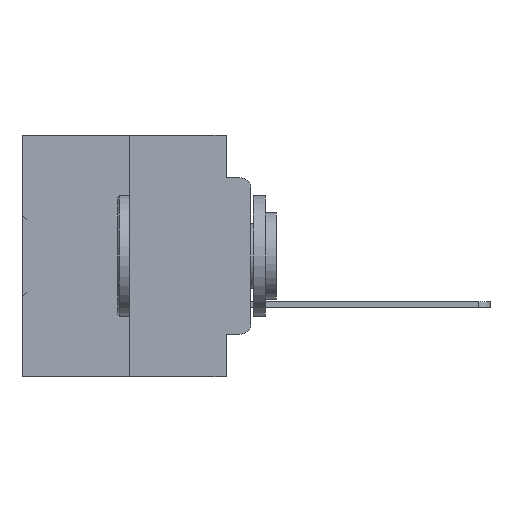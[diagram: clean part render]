
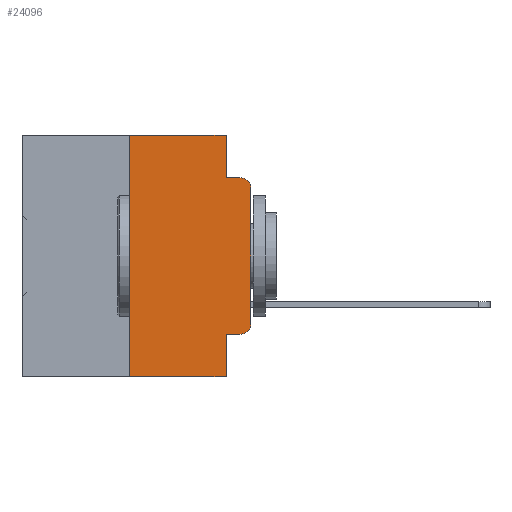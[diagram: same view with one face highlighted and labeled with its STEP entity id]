
A CAD part, left-side view. The second image highlights one B-rep face of the part: STEP entity #24096.
In plain terms, the highlighted planar face has unit normal (-1, 0, 0).
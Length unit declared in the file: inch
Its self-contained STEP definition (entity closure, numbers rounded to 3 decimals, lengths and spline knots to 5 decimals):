
#354 = DIRECTION ( 'NONE',  ( 0., 0., -1. ) ) ;
#585 = ORIENTED_EDGE ( 'NONE', *, *, #23253, .F. ) ;
#699 = EDGE_CURVE ( 'NONE', #13239, #17577, #24076, .T. ) ;
#1765 = ORIENTED_EDGE ( 'NONE', *, *, #35002, .F. ) ;
#1872 = ORIENTED_EDGE ( 'NONE', *, *, #27103, .F. ) ;
#2920 = VERTEX_POINT ( 'NONE', #25099 ) ;
#3272 = ORIENTED_EDGE ( 'NONE', *, *, #11423, .T. ) ;
#3606 = LINE ( 'NONE', #4797, #32485 ) ;
#4033 = CIRCLE ( 'NONE', #13072, 0.02 ) ;
#4127 = ORIENTED_EDGE ( 'NONE', *, *, #17073, .T. ) ;
#4234 = CARTESIAN_POINT ( 'NONE',  ( 0., 0.051, -0.0885 ) ) ;
#4304 = VERTEX_POINT ( 'NONE', #31393 ) ;
#4423 = VERTEX_POINT ( 'NONE', #23908 ) ;
#4560 = CARTESIAN_POINT ( 'NONE',  ( 0., 0.473, 0. ) ) ;
#4667 = VERTEX_POINT ( 'NONE', #35616 ) ;
#4797 = CARTESIAN_POINT ( 'NONE',  ( 0., 0.051, 0. ) ) ;
#4916 = ORIENTED_EDGE ( 'NONE', *, *, #32068, .F. ) ;
#5108 = ORIENTED_EDGE ( 'NONE', *, *, #699, .T. ) ;
#5327 = DIRECTION ( 'NONE',  ( -1., 0., 0. ) ) ;
#6555 = LINE ( 'NONE', #34905, #35234 ) ;
#7969 = CARTESIAN_POINT ( 'NONE',  ( 0., 0.25, -0.5 ) ) ;
#8515 = ORIENTED_EDGE ( 'NONE', *, *, #27800, .F. ) ;
#8553 = CARTESIAN_POINT ( 'NONE',  ( 0., 0.051, 0. ) ) ;
#8704 = CARTESIAN_POINT ( 'NONE',  ( 0., 0.02, -0.3915 ) ) ;
#11055 = DIRECTION ( 'NONE',  ( 0., -1., 0. ) ) ;
#11423 = EDGE_CURVE ( 'NONE', #16137, #4423, #13098, .T. ) ;
#11574 = DIRECTION ( 'NONE',  ( 0., 0., -1. ) ) ;
#11803 = CARTESIAN_POINT ( 'NONE',  ( 0., 0.473, -0.5 ) ) ;
#13072 = AXIS2_PLACEMENT_3D ( 'NONE', #8704, #28272, #11574 ) ;
#13098 = CIRCLE ( 'NONE', #21456, 0.02 ) ;
#13239 = VERTEX_POINT ( 'NONE', #7969 ) ;
#13851 = AXIS2_PLACEMENT_3D ( 'NONE', #25695, #17377, #354 ) ;
#14161 = DIRECTION ( 'NONE',  ( 0., 0., -1. ) ) ;
#15068 = CARTESIAN_POINT ( 'NONE',  ( 0., 0.25, 0. ) ) ;
#15663 = DIRECTION ( 'NONE',  ( 0., 0., 1. ) ) ;
#15731 = VECTOR ( 'NONE', #11055, 39.37008 ) ;
#16137 = VERTEX_POINT ( 'NONE', #26093 ) ;
#16382 = VECTOR ( 'NONE', #24049, 39.37008 ) ;
#16890 = ORIENTED_EDGE ( 'NONE', *, *, #34526, .T. ) ;
#17073 = EDGE_CURVE ( 'NONE', #2920, #16137, #35435, .T. ) ;
#17377 = DIRECTION ( 'NONE',  ( 1., 0., 0. ) ) ;
#17577 = VERTEX_POINT ( 'NONE', #29614 ) ;
#17838 = ORIENTED_EDGE ( 'NONE', *, *, #35220, .T. ) ;
#18851 = DIRECTION ( 'NONE',  ( 0., -1., 0. ) ) ;
#19090 = DIRECTION ( 'NONE',  ( 0., 0., -1. ) ) ;
#19139 = DIRECTION ( 'NONE',  ( 0., 0., 1. ) ) ;
#19426 = VERTEX_POINT ( 'NONE', #15068 ) ;
#20495 = VECTOR ( 'NONE', #33374, 39.37008 ) ;
#21456 = AXIS2_PLACEMENT_3D ( 'NONE', #22257, #5327, #25089 ) ;
#22231 = VECTOR ( 'NONE', #14161, 39.37008 ) ;
#22257 = CARTESIAN_POINT ( 'NONE',  ( 0., 0.02, -0.1085 ) ) ;
#22528 = CARTESIAN_POINT ( 'NONE',  ( 0., 0.051, -0.4115 ) ) ;
#22838 = LINE ( 'NONE', #4560, #28424 ) ;
#23253 = EDGE_CURVE ( 'NONE', #19426, #4667, #22838, .T. ) ;
#23740 = CARTESIAN_POINT ( 'NONE',  ( 0., 0.051, -0.0885 ) ) ;
#23908 = CARTESIAN_POINT ( 'NONE',  ( 0., 0.02, -0.0885 ) ) ;
#24049 = DIRECTION ( 'NONE',  ( 0., -1., 0. ) ) ;
#24076 = LINE ( 'NONE', #11803, #15731 ) ;
#24096 = ADVANCED_FACE ( 'NONE', ( #24387 ), #33835, .F. ) ;
#24387 = FACE_OUTER_BOUND ( 'NONE', #34976, .T. ) ;
#24678 = VERTEX_POINT ( 'NONE', #30876 ) ;
#24693 = LINE ( 'NONE', #4234, #16382 ) ;
#25089 = DIRECTION ( 'NONE',  ( 0., 0., -1. ) ) ;
#25099 = CARTESIAN_POINT ( 'NONE',  ( 0., 0., -0.3915 ) ) ;
#25695 = CARTESIAN_POINT ( 'NONE',  ( 0., 0.473, 0. ) ) ;
#26093 = CARTESIAN_POINT ( 'NONE',  ( 0., 0., -0.1085 ) ) ;
#27103 = EDGE_CURVE ( 'NONE', #29319, #4423, #24693, .T. ) ;
#27800 = EDGE_CURVE ( 'NONE', #13239, #19426, #6555, .T. ) ;
#28268 = VECTOR ( 'NONE', #19139, 39.37008 ) ;
#28272 = DIRECTION ( 'NONE',  ( -1., 0., 0. ) ) ;
#28424 = VECTOR ( 'NONE', #18851, 39.37008 ) ;
#29319 = VERTEX_POINT ( 'NONE', #23740 ) ;
#29614 = CARTESIAN_POINT ( 'NONE',  ( 0., 0.051, -0.5 ) ) ;
#30120 = CARTESIAN_POINT ( 'NONE',  ( 0., 0., 0. ) ) ;
#30409 = LINE ( 'NONE', #8553, #22231 ) ;
#30876 = CARTESIAN_POINT ( 'NONE',  ( 0., 0.02, -0.4115 ) ) ;
#31393 = CARTESIAN_POINT ( 'NONE',  ( 0., 0.051, -0.4115 ) ) ;
#32068 = EDGE_CURVE ( 'NONE', #4304, #17577, #30409, .T. ) ;
#32485 = VECTOR ( 'NONE', #19090, 39.37008 ) ;
#33374 = DIRECTION ( 'NONE',  ( 0., -1., 0. ) ) ;
#33835 = PLANE ( 'NONE',  #13851 ) ;
#34526 = EDGE_CURVE ( 'NONE', #4304, #24678, #35053, .T. ) ;
#34905 = CARTESIAN_POINT ( 'NONE',  ( 0., 0.25, 0. ) ) ;
#34976 = EDGE_LOOP ( 'NONE', ( #4127, #3272, #1872, #1765, #585, #8515, #5108, #4916, #16890, #17838 ) ) ;
#35002 = EDGE_CURVE ( 'NONE', #4667, #29319, #3606, .T. ) ;
#35053 = LINE ( 'NONE', #22528, #20495 ) ;
#35220 = EDGE_CURVE ( 'NONE', #24678, #2920, #4033, .T. ) ;
#35234 = VECTOR ( 'NONE', #15663, 39.37008 ) ;
#35435 = LINE ( 'NONE', #30120, #28268 ) ;
#35616 = CARTESIAN_POINT ( 'NONE',  ( 0., 0.051, 0. ) ) ;
